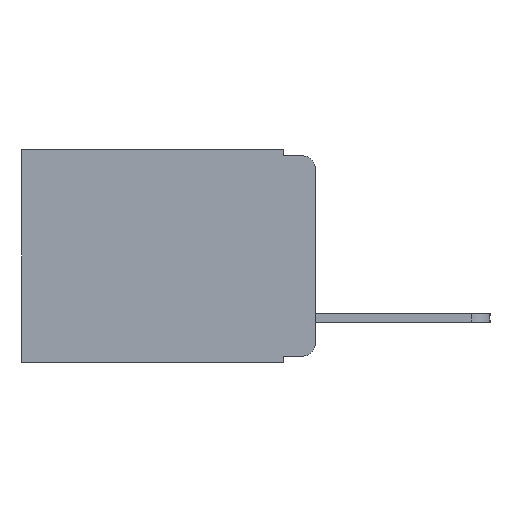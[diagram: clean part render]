
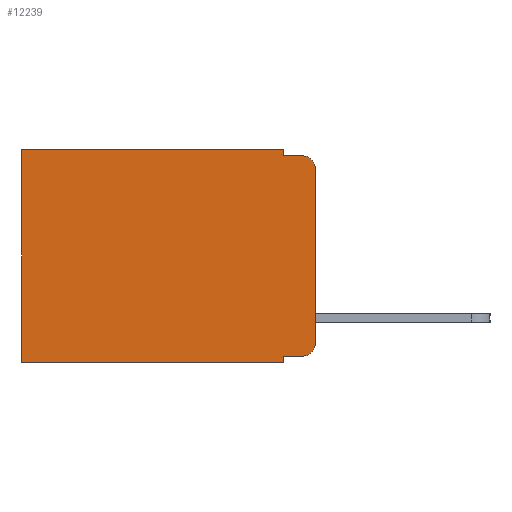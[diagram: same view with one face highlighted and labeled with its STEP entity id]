
A CAD part, left-side view. The second image highlights one B-rep face of the part: STEP entity #12239.
In plain terms, the highlighted planar face has unit normal (-1, 0, 0).
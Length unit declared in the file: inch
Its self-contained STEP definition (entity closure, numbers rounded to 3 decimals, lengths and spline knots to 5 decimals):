
#215 = CARTESIAN_POINT ( 'NONE',  ( 0.298, 0., -0.03 ) ) ;
#390 = ORIENTED_EDGE ( 'NONE', *, *, #4670, .T. ) ;
#955 = ORIENTED_EDGE ( 'NONE', *, *, #3595, .T. ) ;
#1219 = DIRECTION ( 'NONE',  ( 0., -1., 0. ) ) ;
#1247 = EDGE_CURVE ( 'NONE', #13600, #11475, #8516, .T. ) ;
#1348 = CARTESIAN_POINT ( 'NONE',  ( 0.298, 0.051, 0. ) ) ;
#1385 = CARTESIAN_POINT ( 'NONE',  ( 0.298, 0.051, -0.343 ) ) ;
#1733 = PLANE ( 'NONE',  #11758 ) ;
#2234 = ORIENTED_EDGE ( 'NONE', *, *, #10008, .T. ) ;
#2276 = LINE ( 'NONE', #14561, #18180 ) ;
#2736 = DIRECTION ( 'NONE',  ( 0., 0., -1. ) ) ;
#2850 = CARTESIAN_POINT ( 'NONE',  ( 0.298, 0., 0. ) ) ;
#2974 = DIRECTION ( 'NONE',  ( 0., 1., 0. ) ) ;
#3142 = DIRECTION ( 'NONE',  ( 0., -1., 0. ) ) ;
#3417 = DIRECTION ( 'NONE',  ( 0., 0., -1. ) ) ;
#3595 = EDGE_CURVE ( 'NONE', #4716, #3794, #11376, .T. ) ;
#3794 = VERTEX_POINT ( 'NONE', #18556 ) ;
#4126 = VERTEX_POINT ( 'NONE', #1385 ) ;
#4670 = EDGE_CURVE ( 'NONE', #14306, #4716, #13242, .T. ) ;
#4716 = VERTEX_POINT ( 'NONE', #8293 ) ;
#4963 = CARTESIAN_POINT ( 'NONE',  ( 0.298, 0., 0. ) ) ;
#5005 = CARTESIAN_POINT ( 'NONE',  ( 0.298, 0.473, -0.343 ) ) ;
#5534 = VERTEX_POINT ( 'NONE', #19933 ) ;
#5756 = EDGE_CURVE ( 'NONE', #14306, #4126, #10219, .T. ) ;
#5921 = CARTESIAN_POINT ( 'NONE',  ( 0.298, 0.051, 0. ) ) ;
#6806 = EDGE_CURVE ( 'NONE', #11475, #13012, #8642, .T. ) ;
#6855 = CIRCLE ( 'NONE', #18624, 0.02 ) ;
#7030 = CARTESIAN_POINT ( 'NONE',  ( 0.298, 0.051, -0.333 ) ) ;
#7034 = ORIENTED_EDGE ( 'NONE', *, *, #7865, .F. ) ;
#7458 = DIRECTION ( 'NONE',  ( -1., 0., 0. ) ) ;
#7537 = ORIENTED_EDGE ( 'NONE', *, *, #1247, .T. ) ;
#7822 = DIRECTION ( 'NONE',  ( 0., 0., -1. ) ) ;
#7865 = EDGE_CURVE ( 'NONE', #13600, #9793, #15040, .T. ) ;
#7989 = CARTESIAN_POINT ( 'NONE',  ( 0.298, 0.473, 0. ) ) ;
#8093 = CARTESIAN_POINT ( 'NONE',  ( 0.298, 0.051, -0.333 ) ) ;
#8293 = CARTESIAN_POINT ( 'NONE',  ( 0.298, 0.02, -0.333 ) ) ;
#8516 = LINE ( 'NONE', #2850, #16138 ) ;
#8642 = LINE ( 'NONE', #15488, #19658 ) ;
#8928 = EDGE_CURVE ( 'NONE', #9793, #5534, #19406, .T. ) ;
#8954 = CARTESIAN_POINT ( 'NONE',  ( 0.298, 0.02, -0.313 ) ) ;
#9077 = DIRECTION ( 'NONE',  ( 0., 0., -1. ) ) ;
#9457 = DIRECTION ( 'NONE',  ( -1., 0., 0. ) ) ;
#9793 = VERTEX_POINT ( 'NONE', #10085 ) ;
#10008 = EDGE_CURVE ( 'NONE', #20108, #5534, #6855, .T. ) ;
#10049 = CARTESIAN_POINT ( 'NONE',  ( 0.298, 0.051, -0.01 ) ) ;
#10068 = DIRECTION ( 'NONE',  ( 0., 1., 0. ) ) ;
#10085 = CARTESIAN_POINT ( 'NONE',  ( 0.298, 0.051, -0.01 ) ) ;
#10219 = LINE ( 'NONE', #13054, #19705 ) ;
#10746 = DIRECTION ( 'NONE',  ( 0., 0., -1. ) ) ;
#11376 = CIRCLE ( 'NONE', #11642, 0.02 ) ;
#11475 = VERTEX_POINT ( 'NONE', #7989 ) ;
#11642 = AXIS2_PLACEMENT_3D ( 'NONE', #8954, #9457, #10746 ) ;
#11668 = EDGE_CURVE ( 'NONE', #4126, #13012, #2276, .T. ) ;
#11687 = ORIENTED_EDGE ( 'NONE', *, *, #6806, .T. ) ;
#11758 = AXIS2_PLACEMENT_3D ( 'NONE', #4963, #12851, #3417 ) ;
#12069 = EDGE_CURVE ( 'NONE', #20108, #3794, #19220, .T. ) ;
#12239 = ADVANCED_FACE ( 'NONE', ( #17412 ), #1733, .F. ) ;
#12851 = DIRECTION ( 'NONE',  ( 1., 0., 0. ) ) ;
#13012 = VERTEX_POINT ( 'NONE', #5005 ) ;
#13054 = CARTESIAN_POINT ( 'NONE',  ( 0.298, 0.051, 0. ) ) ;
#13242 = LINE ( 'NONE', #7030, #16685 ) ;
#13600 = VERTEX_POINT ( 'NONE', #1348 ) ;
#13974 = CARTESIAN_POINT ( 'NONE',  ( 0.298, 0., 0. ) ) ;
#14306 = VERTEX_POINT ( 'NONE', #8093 ) ;
#14561 = CARTESIAN_POINT ( 'NONE',  ( 0.298, 0., -0.343 ) ) ;
#14735 = ORIENTED_EDGE ( 'NONE', *, *, #8928, .F. ) ;
#14982 = EDGE_LOOP ( 'NONE', ( #18149, #2234, #14735, #7034, #7537, #11687, #16129, #16571, #390, #955 ) ) ;
#15040 = LINE ( 'NONE', #5921, #18436 ) ;
#15071 = VECTOR ( 'NONE', #3142, 39.37008 ) ;
#15352 = VECTOR ( 'NONE', #7822, 39.37008 ) ;
#15488 = CARTESIAN_POINT ( 'NONE',  ( 0.298, 0.473, 0. ) ) ;
#15846 = DIRECTION ( 'NONE',  ( 0., 0., -1. ) ) ;
#16129 = ORIENTED_EDGE ( 'NONE', *, *, #11668, .F. ) ;
#16138 = VECTOR ( 'NONE', #2974, 39.37008 ) ;
#16556 = CARTESIAN_POINT ( 'NONE',  ( 0.298, 0.02, -0.03 ) ) ;
#16571 = ORIENTED_EDGE ( 'NONE', *, *, #5756, .F. ) ;
#16685 = VECTOR ( 'NONE', #1219, 39.37008 ) ;
#17412 = FACE_OUTER_BOUND ( 'NONE', #14982, .T. ) ;
#18024 = DIRECTION ( 'NONE',  ( 0., 0., -1. ) ) ;
#18149 = ORIENTED_EDGE ( 'NONE', *, *, #12069, .F. ) ;
#18180 = VECTOR ( 'NONE', #10068, 39.37008 ) ;
#18436 = VECTOR ( 'NONE', #2736, 39.37008 ) ;
#18556 = CARTESIAN_POINT ( 'NONE',  ( 0.298, 0., -0.313 ) ) ;
#18624 = AXIS2_PLACEMENT_3D ( 'NONE', #16556, #7458, #18024 ) ;
#19220 = LINE ( 'NONE', #13974, #15352 ) ;
#19406 = LINE ( 'NONE', #10049, #15071 ) ;
#19658 = VECTOR ( 'NONE', #9077, 39.37008 ) ;
#19705 = VECTOR ( 'NONE', #15846, 39.37008 ) ;
#19933 = CARTESIAN_POINT ( 'NONE',  ( 0.298, 0.02, -0.01 ) ) ;
#20108 = VERTEX_POINT ( 'NONE', #215 ) ;
